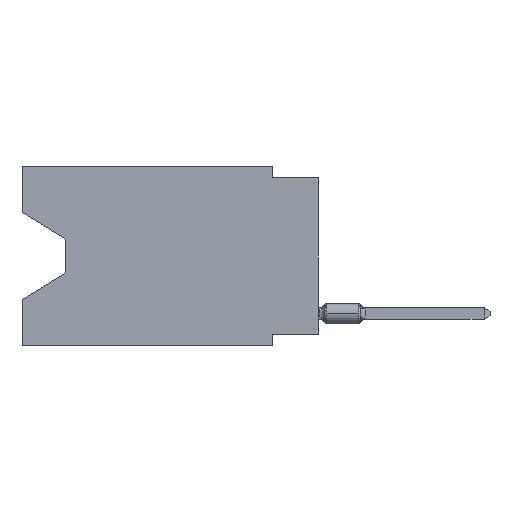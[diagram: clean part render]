
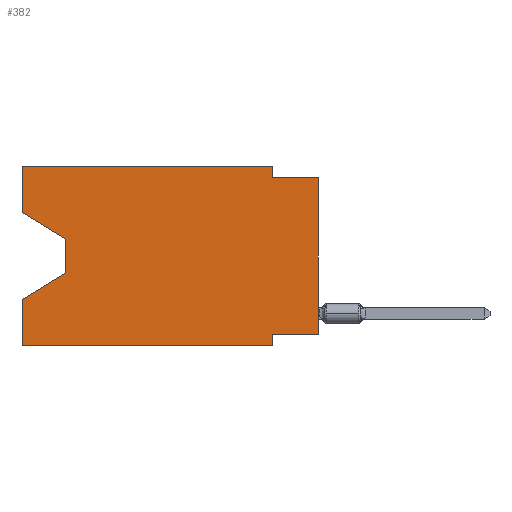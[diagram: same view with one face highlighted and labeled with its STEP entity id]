
A CAD part, left-side view. The second image highlights one B-rep face of the part: STEP entity #382.
In plain terms, the highlighted planar face has unit normal (-1, 0, 0).
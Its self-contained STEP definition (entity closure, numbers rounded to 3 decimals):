
#217 = EDGE_CURVE ( 'NONE', #831, #5833, #12804, .T. ) ;
#382 = ADVANCED_FACE ( 'NONE', ( #5911 ), #14974, .F. ) ;
#790 = LINE ( 'NONE', #6842, #18715 ) ;
#831 = VERTEX_POINT ( 'NONE', #16293 ) ;
#1051 = DIRECTION ( 'NONE',  ( 0., 0., 1. ) ) ;
#1070 = CARTESIAN_POINT ( 'NONE',  ( 0., 16.383, -7.36 ) ) ;
#1235 = VERTEX_POINT ( 'NONE', #13460 ) ;
#1359 = VERTEX_POINT ( 'NONE', #17320 ) ;
#1443 = CARTESIAN_POINT ( 'NONE',  ( 0., 0., -9.271 ) ) ;
#2164 = EDGE_CURVE ( 'NONE', #19012, #5833, #17808, .T. ) ;
#2172 = ORIENTED_EDGE ( 'NONE', *, *, #13775, .F. ) ;
#2219 = VECTOR ( 'NONE', #15156, 1000. ) ;
#2592 = CARTESIAN_POINT ( 'NONE',  ( 0., 16.383, 0. ) ) ;
#2608 = LINE ( 'NONE', #16417, #13674 ) ;
#3268 = LINE ( 'NONE', #6433, #5984 ) ;
#3300 = EDGE_CURVE ( 'NONE', #19344, #10622, #18410, .T. ) ;
#3917 = DIRECTION ( 'NONE',  ( 0., 0.855, -0.519 ) ) ;
#3973 = ORIENTED_EDGE ( 'NONE', *, *, #17916, .F. ) ;
#3981 = ORIENTED_EDGE ( 'NONE', *, *, #2164, .F. ) ;
#4005 = CARTESIAN_POINT ( 'NONE',  ( 0., 13.97, -5.893 ) ) ;
#4781 = DIRECTION ( 'NONE',  ( 0., 0., 1. ) ) ;
#5533 = CARTESIAN_POINT ( 'NONE',  ( 0., 0., -0.635 ) ) ;
#5833 = VERTEX_POINT ( 'NONE', #19018 ) ;
#5911 = FACE_OUTER_BOUND ( 'NONE', #7647, .T. ) ;
#5984 = VECTOR ( 'NONE', #13722, 1000. ) ;
#6071 = CARTESIAN_POINT ( 'NONE',  ( 0., 2.54, 0. ) ) ;
#6082 = VECTOR ( 'NONE', #16218, 1000. ) ;
#6433 = CARTESIAN_POINT ( 'NONE',  ( 0., 16.383, -2.546 ) ) ;
#6554 = LINE ( 'NONE', #12357, #19071 ) ;
#6720 = CARTESIAN_POINT ( 'NONE',  ( 0., 0., -0.635 ) ) ;
#6734 = CARTESIAN_POINT ( 'NONE',  ( 0., 13.97, -5.893 ) ) ;
#6775 = ORIENTED_EDGE ( 'NONE', *, *, #12308, .T. ) ;
#6842 = CARTESIAN_POINT ( 'NONE',  ( 0., 13.97, -4.013 ) ) ;
#6899 = CARTESIAN_POINT ( 'NONE',  ( 0., 16.383, 0. ) ) ;
#7066 = DIRECTION ( 'NONE',  ( 0., 0., -1. ) ) ;
#7288 = VECTOR ( 'NONE', #7066, 1000. ) ;
#7484 = ORIENTED_EDGE ( 'NONE', *, *, #17081, .F. ) ;
#7647 = EDGE_LOOP ( 'NONE', ( #13583, #19528, #6775, #9635, #19632, #3981, #8497, #19320, #3973, #2172, #16091, #7484 ) ) ;
#7909 = VERTEX_POINT ( 'NONE', #1070 ) ;
#8497 = ORIENTED_EDGE ( 'NONE', *, *, #15757, .F. ) ;
#8712 = CARTESIAN_POINT ( 'NONE',  ( 0., 16.383, 0. ) ) ;
#9498 = CARTESIAN_POINT ( 'NONE',  ( 0., 16.383, 0. ) ) ;
#9635 = ORIENTED_EDGE ( 'NONE', *, *, #14789, .F. ) ;
#9874 = VECTOR ( 'NONE', #1051, 1000. ) ;
#9948 = VERTEX_POINT ( 'NONE', #6071 ) ;
#10405 = VERTEX_POINT ( 'NONE', #12023 ) ;
#10568 = CARTESIAN_POINT ( 'NONE',  ( 0., 0., 0. ) ) ;
#10622 = VERTEX_POINT ( 'NONE', #5533 ) ;
#11403 = CARTESIAN_POINT ( 'NONE',  ( 0., 2.54, -9.271 ) ) ;
#11487 = LINE ( 'NONE', #4005, #13951 ) ;
#11507 = DIRECTION ( 'NONE',  ( 0., -1., 0. ) ) ;
#12023 = CARTESIAN_POINT ( 'NONE',  ( 0., 13.97, -4.013 ) ) ;
#12308 = EDGE_CURVE ( 'NONE', #12883, #7909, #11487, .T. ) ;
#12357 = CARTESIAN_POINT ( 'NONE',  ( 0., 0., -9.271 ) ) ;
#12731 = EDGE_CURVE ( 'NONE', #1359, #10405, #3268, .T. ) ;
#12804 = LINE ( 'NONE', #14488, #13387 ) ;
#12883 = VERTEX_POINT ( 'NONE', #6734 ) ;
#12987 = DIRECTION ( 'NONE',  ( 0., -1., 0. ) ) ;
#13264 = LINE ( 'NONE', #18140, #2219 ) ;
#13387 = VECTOR ( 'NONE', #12987, 1000. ) ;
#13460 = CARTESIAN_POINT ( 'NONE',  ( 0., 2.54, -0.635 ) ) ;
#13583 = ORIENTED_EDGE ( 'NONE', *, *, #12731, .T. ) ;
#13674 = VECTOR ( 'NONE', #16630, 1000. ) ;
#13722 = DIRECTION ( 'NONE',  ( 0., -0.855, -0.519 ) ) ;
#13775 = EDGE_CURVE ( 'NONE', #9948, #1235, #13264, .T. ) ;
#13871 = VECTOR ( 'NONE', #4781, 1000. ) ;
#13951 = VECTOR ( 'NONE', #3917, 1000. ) ;
#14044 = DIRECTION ( 'NONE',  ( 0., 1., 0. ) ) ;
#14183 = EDGE_CURVE ( 'NONE', #15387, #9948, #2608, .T. ) ;
#14285 = LINE ( 'NONE', #6720, #18084 ) ;
#14488 = CARTESIAN_POINT ( 'NONE',  ( 0., 16.383, -9.906 ) ) ;
#14779 = DIRECTION ( 'NONE',  ( 1., 0., 0. ) ) ;
#14789 = EDGE_CURVE ( 'NONE', #831, #7909, #17354, .T. ) ;
#14974 = PLANE ( 'NONE',  #14994 ) ;
#14994 = AXIS2_PLACEMENT_3D ( 'NONE', #8712, #14779, #17958 ) ;
#15156 = DIRECTION ( 'NONE',  ( 0., 0., -1. ) ) ;
#15387 = VERTEX_POINT ( 'NONE', #9498 ) ;
#15757 = EDGE_CURVE ( 'NONE', #19344, #19012, #6554, .T. ) ;
#16091 = ORIENTED_EDGE ( 'NONE', *, *, #14183, .F. ) ;
#16114 = LINE ( 'NONE', #2592, #6082 ) ;
#16218 = DIRECTION ( 'NONE',  ( 0., 0., 1. ) ) ;
#16293 = CARTESIAN_POINT ( 'NONE',  ( 0., 16.383, -9.906 ) ) ;
#16417 = CARTESIAN_POINT ( 'NONE',  ( 0., 16.383, 0. ) ) ;
#16630 = DIRECTION ( 'NONE',  ( 0., -1., 0. ) ) ;
#17081 = EDGE_CURVE ( 'NONE', #1359, #15387, #16114, .T. ) ;
#17320 = CARTESIAN_POINT ( 'NONE',  ( 0., 16.383, -2.546 ) ) ;
#17354 = LINE ( 'NONE', #6899, #9874 ) ;
#17405 = CARTESIAN_POINT ( 'NONE',  ( 0., 2.54, -9.906 ) ) ;
#17411 = EDGE_CURVE ( 'NONE', #10405, #12883, #790, .T. ) ;
#17808 = LINE ( 'NONE', #17405, #7288 ) ;
#17916 = EDGE_CURVE ( 'NONE', #1235, #10622, #14285, .T. ) ;
#17958 = DIRECTION ( 'NONE',  ( 0., 0., -1. ) ) ;
#18084 = VECTOR ( 'NONE', #11507, 1000. ) ;
#18140 = CARTESIAN_POINT ( 'NONE',  ( 0., 2.54, 0. ) ) ;
#18410 = LINE ( 'NONE', #10568, #13871 ) ;
#18715 = VECTOR ( 'NONE', #19174, 1000. ) ;
#19012 = VERTEX_POINT ( 'NONE', #11403 ) ;
#19018 = CARTESIAN_POINT ( 'NONE',  ( 0., 2.54, -9.906 ) ) ;
#19071 = VECTOR ( 'NONE', #14044, 1000. ) ;
#19174 = DIRECTION ( 'NONE',  ( 0., 0., -1. ) ) ;
#19320 = ORIENTED_EDGE ( 'NONE', *, *, #3300, .T. ) ;
#19344 = VERTEX_POINT ( 'NONE', #1443 ) ;
#19528 = ORIENTED_EDGE ( 'NONE', *, *, #17411, .T. ) ;
#19632 = ORIENTED_EDGE ( 'NONE', *, *, #217, .T. ) ;
